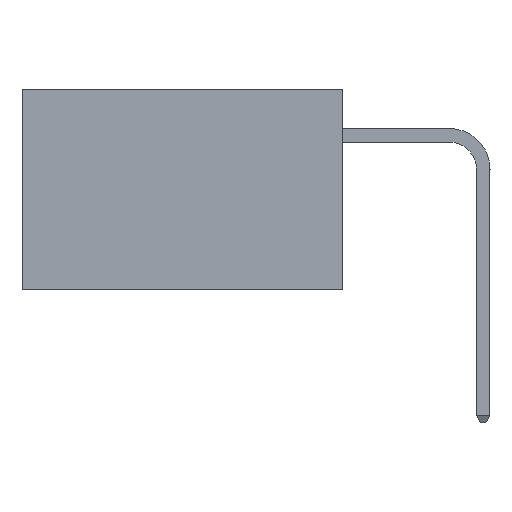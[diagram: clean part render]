
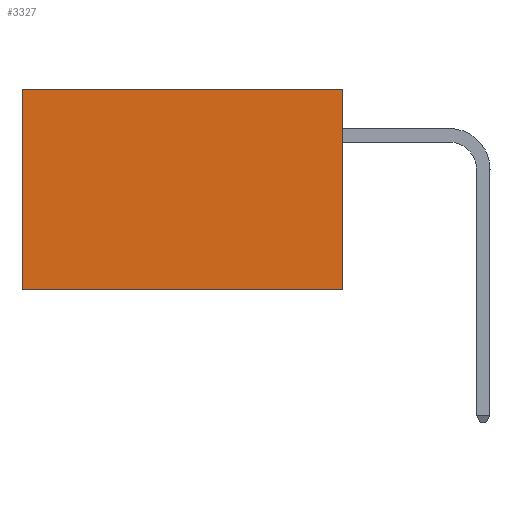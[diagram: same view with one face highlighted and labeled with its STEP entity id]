
A CAD part, left-side view. The second image highlights one B-rep face of the part: STEP entity #3327.
In plain terms, the highlighted planar face has unit normal (-1, 0, 0).
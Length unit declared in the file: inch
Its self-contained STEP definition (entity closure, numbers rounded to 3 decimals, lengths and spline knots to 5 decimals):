
#2162 = VECTOR ( 'NONE', #25310, 39.37008 ) ;
#2537 = PLANE ( 'NONE',  #24737 ) ;
#2591 = CARTESIAN_POINT ( 'NONE',  ( 0.277, 0., -0.37 ) ) ;
#2673 = VERTEX_POINT ( 'NONE', #18216 ) ;
#2741 = ORIENTED_EDGE ( 'NONE', *, *, #7589, .T. ) ;
#3277 = CARTESIAN_POINT ( 'NONE',  ( 0.277, 0.59, 0. ) ) ;
#3327 = ADVANCED_FACE ( 'NONE', ( #21570 ), #2537, .F. ) ;
#4273 = DIRECTION ( 'NONE',  ( 0., 0., -1. ) ) ;
#4736 = DIRECTION ( 'NONE',  ( 1., 0., 0. ) ) ;
#5530 = VECTOR ( 'NONE', #22245, 39.37008 ) ;
#7589 = EDGE_CURVE ( 'NONE', #8143, #15412, #8926, .T. ) ;
#8143 = VERTEX_POINT ( 'NONE', #12868 ) ;
#8926 = LINE ( 'NONE', #30253, #21163 ) ;
#12040 = LINE ( 'NONE', #2591, #5530 ) ;
#12216 = DIRECTION ( 'NONE',  ( 0., 0., -1. ) ) ;
#12868 = CARTESIAN_POINT ( 'NONE',  ( 0.277, 0., 0. ) ) ;
#13558 = CARTESIAN_POINT ( 'NONE',  ( 0.277, 0., -0.37 ) ) ;
#14288 = ORIENTED_EDGE ( 'NONE', *, *, #26707, .F. ) ;
#15056 = ORIENTED_EDGE ( 'NONE', *, *, #20023, .F. ) ;
#15412 = VERTEX_POINT ( 'NONE', #3277 ) ;
#16589 = EDGE_CURVE ( 'NONE', #15412, #2673, #23389, .T. ) ;
#18216 = CARTESIAN_POINT ( 'NONE',  ( 0.277, 0.59, -0.37 ) ) ;
#18251 = DIRECTION ( 'NONE',  ( 0., 1., 0. ) ) ;
#20023 = EDGE_CURVE ( 'NONE', #8143, #30665, #21016, .T. ) ;
#21016 = LINE ( 'NONE', #22916, #2162 ) ;
#21163 = VECTOR ( 'NONE', #18251, 39.37008 ) ;
#21570 = FACE_OUTER_BOUND ( 'NONE', #22761, .T. ) ;
#22245 = DIRECTION ( 'NONE',  ( 0., 1., 0. ) ) ;
#22761 = EDGE_LOOP ( 'NONE', ( #30532, #14288, #15056, #2741 ) ) ;
#22916 = CARTESIAN_POINT ( 'NONE',  ( 0.277, 0., -0.37 ) ) ;
#23389 = LINE ( 'NONE', #24388, #29741 ) ;
#24388 = CARTESIAN_POINT ( 'NONE',  ( 0.277, 0.59, -0.37 ) ) ;
#24737 = AXIS2_PLACEMENT_3D ( 'NONE', #29941, #4736, #4273 ) ;
#25310 = DIRECTION ( 'NONE',  ( 0., 0., -1. ) ) ;
#26707 = EDGE_CURVE ( 'NONE', #30665, #2673, #12040, .T. ) ;
#29741 = VECTOR ( 'NONE', #12216, 39.37008 ) ;
#29941 = CARTESIAN_POINT ( 'NONE',  ( 0.277, 0., -0.37 ) ) ;
#30253 = CARTESIAN_POINT ( 'NONE',  ( 0.277, 0., 0. ) ) ;
#30532 = ORIENTED_EDGE ( 'NONE', *, *, #16589, .T. ) ;
#30665 = VERTEX_POINT ( 'NONE', #13558 ) ;
